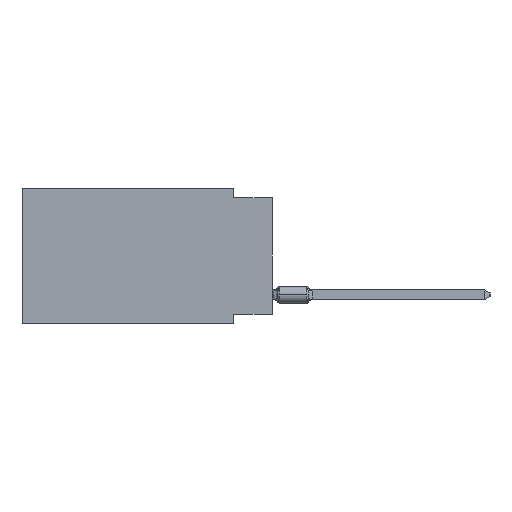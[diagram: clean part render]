
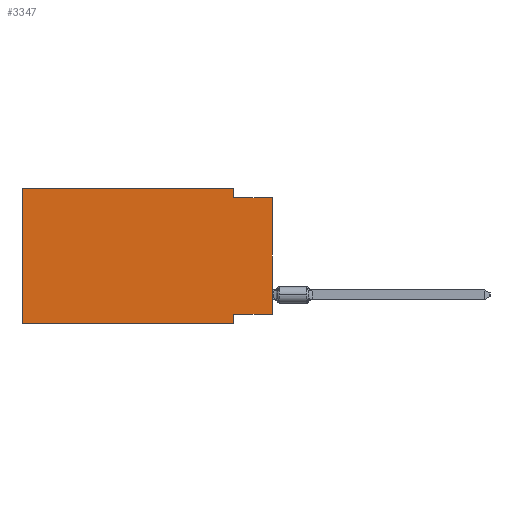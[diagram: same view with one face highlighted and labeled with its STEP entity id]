
A CAD part, left-side view. The second image highlights one B-rep face of the part: STEP entity #3347.
In plain terms, the highlighted planar face has unit normal (-1, 0, 0).
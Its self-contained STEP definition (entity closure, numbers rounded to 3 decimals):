
#194 = AXIS2_PLACEMENT_3D ( 'NONE', #22875, #28298, #17959 ) ;
#1549 = DIRECTION ( 'NONE',  ( 0., -1., 0. ) ) ;
#1879 = LINE ( 'NONE', #17016, #1931 ) ;
#1907 = CARTESIAN_POINT ( 'NONE',  ( 0., 0., -0.635 ) ) ;
#1931 = VECTOR ( 'NONE', #1549, 1000. ) ;
#2141 = CARTESIAN_POINT ( 'NONE',  ( 0., 16.383, 0. ) ) ;
#2151 = ORIENTED_EDGE ( 'NONE', *, *, #10809, .F. ) ;
#2207 = CARTESIAN_POINT ( 'NONE',  ( 0., 0., -8.255 ) ) ;
#2549 = ORIENTED_EDGE ( 'NONE', *, *, #26382, .F. ) ;
#2651 = DIRECTION ( 'NONE',  ( 0., -1., 0. ) ) ;
#3347 = ADVANCED_FACE ( 'NONE', ( #20314 ), #4703, .F. ) ;
#3776 = CARTESIAN_POINT ( 'NONE',  ( 0., 2.54, -0.635 ) ) ;
#4098 = EDGE_CURVE ( 'NONE', #21450, #8174, #17895, .T. ) ;
#4703 = PLANE ( 'NONE',  #194 ) ;
#4848 = EDGE_CURVE ( 'NONE', #27208, #26838, #33551, .T. ) ;
#4953 = EDGE_CURVE ( 'NONE', #27208, #30362, #30824, .T. ) ;
#5692 = VECTOR ( 'NONE', #2651, 1000. ) ;
#5722 = ORIENTED_EDGE ( 'NONE', *, *, #4953, .T. ) ;
#6267 = CARTESIAN_POINT ( 'NONE',  ( 0., 16.383, -8.89 ) ) ;
#6778 = VECTOR ( 'NONE', #30492, 1000. ) ;
#6971 = ORIENTED_EDGE ( 'NONE', *, *, #4848, .F. ) ;
#7083 = CARTESIAN_POINT ( 'NONE',  ( 0., 2.54, 0. ) ) ;
#8122 = EDGE_LOOP ( 'NONE', ( #30000, #31082, #20701, #2549, #6971, #5722, #21224, #2151 ) ) ;
#8174 = VERTEX_POINT ( 'NONE', #1907 ) ;
#10809 = EDGE_CURVE ( 'NONE', #21450, #11983, #22929, .T. ) ;
#11194 = EDGE_CURVE ( 'NONE', #25117, #8174, #15165, .T. ) ;
#11224 = VECTOR ( 'NONE', #13587, 1000. ) ;
#11908 = CARTESIAN_POINT ( 'NONE',  ( 0., 16.383, 0. ) ) ;
#11983 = VERTEX_POINT ( 'NONE', #21452 ) ;
#12582 = DIRECTION ( 'NONE',  ( 0., 1., 0. ) ) ;
#13183 = CARTESIAN_POINT ( 'NONE',  ( 0., 0., -8.255 ) ) ;
#13587 = DIRECTION ( 'NONE',  ( 0., 0., -1. ) ) ;
#15165 = LINE ( 'NONE', #33480, #21141 ) ;
#15332 = DIRECTION ( 'NONE',  ( 0., -1., 0. ) ) ;
#16395 = CARTESIAN_POINT ( 'NONE',  ( 0., 2.54, 0. ) ) ;
#17016 = CARTESIAN_POINT ( 'NONE',  ( 0., 16.383, 0. ) ) ;
#17402 = DIRECTION ( 'NONE',  ( 0., 0., 1. ) ) ;
#17895 = LINE ( 'NONE', #30778, #20281 ) ;
#17959 = DIRECTION ( 'NONE',  ( 0., 0., -1. ) ) ;
#18388 = EDGE_CURVE ( 'NONE', #11983, #30362, #21883, .T. ) ;
#20281 = VECTOR ( 'NONE', #17402, 1000. ) ;
#20314 = FACE_OUTER_BOUND ( 'NONE', #8122, .T. ) ;
#20641 = LINE ( 'NONE', #7083, #23262 ) ;
#20701 = ORIENTED_EDGE ( 'NONE', *, *, #23532, .F. ) ;
#21141 = VECTOR ( 'NONE', #15332, 1000. ) ;
#21224 = ORIENTED_EDGE ( 'NONE', *, *, #18388, .F. ) ;
#21450 = VERTEX_POINT ( 'NONE', #13183 ) ;
#21452 = CARTESIAN_POINT ( 'NONE',  ( 0., 2.54, -8.255 ) ) ;
#21883 = LINE ( 'NONE', #32239, #11224 ) ;
#22339 = CARTESIAN_POINT ( 'NONE',  ( 0., 2.54, -8.89 ) ) ;
#22875 = CARTESIAN_POINT ( 'NONE',  ( 0., 16.383, 0. ) ) ;
#22929 = LINE ( 'NONE', #2207, #23871 ) ;
#23203 = DIRECTION ( 'NONE',  ( 0., 0., -1. ) ) ;
#23206 = CARTESIAN_POINT ( 'NONE',  ( 0., 16.383, -8.89 ) ) ;
#23262 = VECTOR ( 'NONE', #23203, 1000. ) ;
#23532 = EDGE_CURVE ( 'NONE', #30250, #25117, #20641, .T. ) ;
#23871 = VECTOR ( 'NONE', #12582, 1000. ) ;
#25117 = VERTEX_POINT ( 'NONE', #3776 ) ;
#26382 = EDGE_CURVE ( 'NONE', #26838, #30250, #1879, .T. ) ;
#26838 = VERTEX_POINT ( 'NONE', #11908 ) ;
#27208 = VERTEX_POINT ( 'NONE', #6267 ) ;
#28298 = DIRECTION ( 'NONE',  ( 1., 0., 0. ) ) ;
#30000 = ORIENTED_EDGE ( 'NONE', *, *, #4098, .T. ) ;
#30250 = VERTEX_POINT ( 'NONE', #16395 ) ;
#30362 = VERTEX_POINT ( 'NONE', #22339 ) ;
#30492 = DIRECTION ( 'NONE',  ( 0., 0., 1. ) ) ;
#30778 = CARTESIAN_POINT ( 'NONE',  ( 0., 0., 0. ) ) ;
#30824 = LINE ( 'NONE', #23206, #5692 ) ;
#31082 = ORIENTED_EDGE ( 'NONE', *, *, #11194, .F. ) ;
#32239 = CARTESIAN_POINT ( 'NONE',  ( 0., 2.54, -8.89 ) ) ;
#33480 = CARTESIAN_POINT ( 'NONE',  ( 0., 0., -0.635 ) ) ;
#33551 = LINE ( 'NONE', #2141, #6778 ) ;
